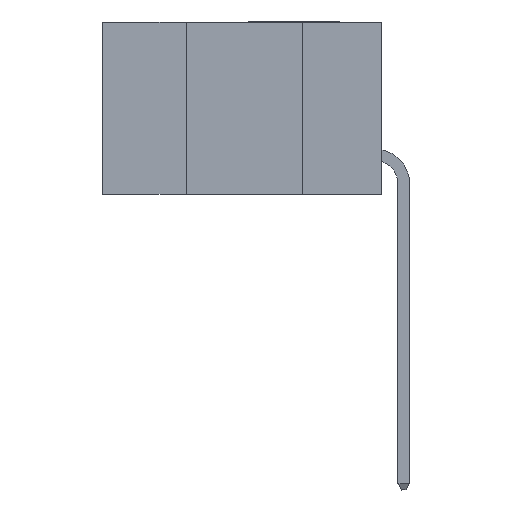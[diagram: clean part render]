
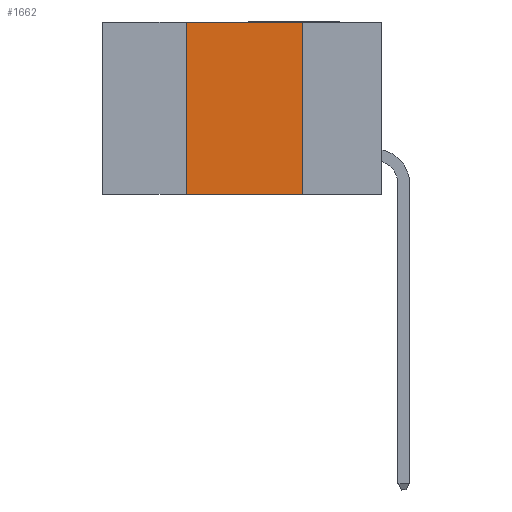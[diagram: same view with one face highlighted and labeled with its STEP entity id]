
A CAD part, left-side view. The second image highlights one B-rep face of the part: STEP entity #1662.
In plain terms, the highlighted planar face has unit normal (-1, 0, 0).
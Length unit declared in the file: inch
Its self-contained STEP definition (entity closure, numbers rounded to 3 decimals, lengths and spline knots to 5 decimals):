
#431 = FACE_OUTER_BOUND ( 'NONE', #6432, .T. ) ;
#455 = CARTESIAN_POINT ( 'NONE',  ( 0., 0.42, 0. ) ) ;
#605 = LINE ( 'NONE', #5330, #6911 ) ;
#730 = DIRECTION ( 'NONE',  ( 0., 0., 1. ) ) ;
#758 = ORIENTED_EDGE ( 'NONE', *, *, #4054, .F. ) ;
#882 = AXIS2_PLACEMENT_3D ( 'NONE', #8585, #2938, #2970 ) ;
#1182 = DIRECTION ( 'NONE',  ( 0., -1., 0. ) ) ;
#1375 = CARTESIAN_POINT ( 'NONE',  ( 0., 0.42, 0. ) ) ;
#1522 = DIRECTION ( 'NONE',  ( 0., -1., 0. ) ) ;
#1530 = ORIENTED_EDGE ( 'NONE', *, *, #7893, .T. ) ;
#1662 = ADVANCED_FACE ( 'NONE', ( #431 ), #2251, .F. ) ;
#1693 = VECTOR ( 'NONE', #730, 39.37008 ) ;
#2251 = PLANE ( 'NONE',  #882 ) ;
#2274 = ORIENTED_EDGE ( 'NONE', *, *, #3413, .F. ) ;
#2884 = VECTOR ( 'NONE', #5321, 39.37008 ) ;
#2938 = DIRECTION ( 'NONE',  ( 1., 0., 0. ) ) ;
#2970 = DIRECTION ( 'NONE',  ( 0., 0., -1. ) ) ;
#3324 = VERTEX_POINT ( 'NONE', #3737 ) ;
#3413 = EDGE_CURVE ( 'NONE', #6878, #4893, #605, .T. ) ;
#3737 = CARTESIAN_POINT ( 'NONE',  ( 0., 0.42, -0.37 ) ) ;
#4054 = EDGE_CURVE ( 'NONE', #3324, #6878, #7228, .T. ) ;
#4195 = LINE ( 'NONE', #6564, #8553 ) ;
#4893 = VERTEX_POINT ( 'NONE', #8503 ) ;
#5321 = DIRECTION ( 'NONE',  ( 0., 0., -1. ) ) ;
#5330 = CARTESIAN_POINT ( 'NONE',  ( 0., 0.6, 0. ) ) ;
#6432 = EDGE_LOOP ( 'NONE', ( #7095, #2274, #758, #1530 ) ) ;
#6564 = CARTESIAN_POINT ( 'NONE',  ( 0., 0.6, -0.37 ) ) ;
#6703 = CARTESIAN_POINT ( 'NONE',  ( 0., 0.17, -0.37 ) ) ;
#6878 = VERTEX_POINT ( 'NONE', #455 ) ;
#6911 = VECTOR ( 'NONE', #1182, 39.37008 ) ;
#7095 = ORIENTED_EDGE ( 'NONE', *, *, #8832, .F. ) ;
#7228 = LINE ( 'NONE', #1375, #1693 ) ;
#7893 = EDGE_CURVE ( 'NONE', #3324, #8562, #4195, .T. ) ;
#8503 = CARTESIAN_POINT ( 'NONE',  ( 0., 0.17, 0. ) ) ;
#8553 = VECTOR ( 'NONE', #1522, 39.37008 ) ;
#8562 = VERTEX_POINT ( 'NONE', #6703 ) ;
#8585 = CARTESIAN_POINT ( 'NONE',  ( 0., 0.6, 0. ) ) ;
#8678 = CARTESIAN_POINT ( 'NONE',  ( 0., 0.17, 0. ) ) ;
#8832 = EDGE_CURVE ( 'NONE', #4893, #8562, #8957, .T. ) ;
#8957 = LINE ( 'NONE', #8678, #2884 ) ;
